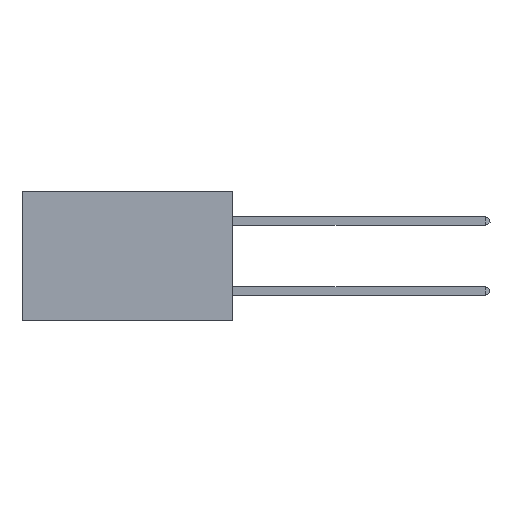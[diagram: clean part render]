
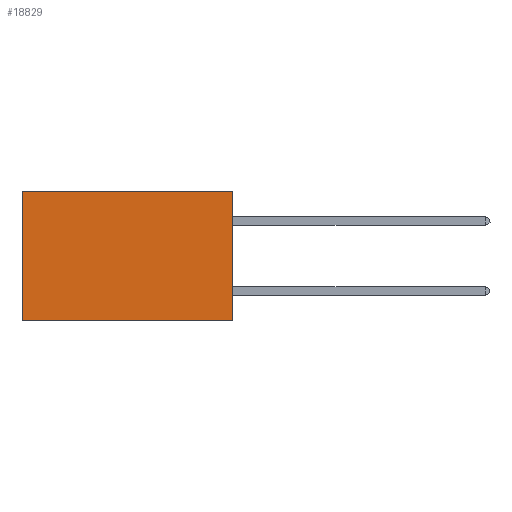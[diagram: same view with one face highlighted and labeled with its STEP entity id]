
A CAD part, left-side view. The second image highlights one B-rep face of the part: STEP entity #18829.
In plain terms, the highlighted planar face has unit normal (-1, 0, 0).
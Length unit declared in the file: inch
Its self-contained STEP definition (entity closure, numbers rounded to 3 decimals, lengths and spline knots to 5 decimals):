
#159 = AXIS2_PLACEMENT_3D ( 'NONE', #17893, #19442, #7616 ) ;
#1968 = LINE ( 'NONE', #11801, #20362 ) ;
#3338 = EDGE_CURVE ( 'NONE', #8968, #4471, #14071, .T. ) ;
#4471 = VERTEX_POINT ( 'NONE', #11150 ) ;
#4704 = DIRECTION ( 'NONE',  ( 0., 0., -1. ) ) ;
#5251 = ORIENTED_EDGE ( 'NONE', *, *, #19631, .T. ) ;
#5755 = ORIENTED_EDGE ( 'NONE', *, *, #20566, .F. ) ;
#6008 = PLANE ( 'NONE',  #159 ) ;
#6185 = CARTESIAN_POINT ( 'NONE',  ( 0.2875, 0., 0. ) ) ;
#6643 = CARTESIAN_POINT ( 'NONE',  ( 0.2875, 0., -0.37 ) ) ;
#6672 = DIRECTION ( 'NONE',  ( 0., 0., -1. ) ) ;
#6883 = VECTOR ( 'NONE', #18465, 39.37008 ) ;
#7099 = ORIENTED_EDGE ( 'NONE', *, *, #9018, .T. ) ;
#7616 = DIRECTION ( 'NONE',  ( 0., 0., -1. ) ) ;
#7889 = CARTESIAN_POINT ( 'NONE',  ( 0.2875, 0.6, 0. ) ) ;
#7959 = VERTEX_POINT ( 'NONE', #7889 ) ;
#7992 = LINE ( 'NONE', #21994, #21029 ) ;
#8968 = VERTEX_POINT ( 'NONE', #10997 ) ;
#9018 = EDGE_CURVE ( 'NONE', #7959, #4471, #7992, .T. ) ;
#10997 = CARTESIAN_POINT ( 'NONE',  ( 0.2875, 0., -0.37 ) ) ;
#11150 = CARTESIAN_POINT ( 'NONE',  ( 0.2875, 0.6, -0.37 ) ) ;
#11801 = CARTESIAN_POINT ( 'NONE',  ( 0.2875, 0., 0. ) ) ;
#12935 = VECTOR ( 'NONE', #21200, 39.37008 ) ;
#14071 = LINE ( 'NONE', #6643, #6883 ) ;
#14883 = FACE_OUTER_BOUND ( 'NONE', #21826, .T. ) ;
#15905 = CARTESIAN_POINT ( 'NONE',  ( 0.2875, 0., 0. ) ) ;
#17784 = LINE ( 'NONE', #15905, #12935 ) ;
#17893 = CARTESIAN_POINT ( 'NONE',  ( 0.2875, 0., 0. ) ) ;
#18003 = ORIENTED_EDGE ( 'NONE', *, *, #3338, .F. ) ;
#18306 = VERTEX_POINT ( 'NONE', #6185 ) ;
#18465 = DIRECTION ( 'NONE',  ( 0., 1., 0. ) ) ;
#18829 = ADVANCED_FACE ( 'NONE', ( #14883 ), #6008, .F. ) ;
#19442 = DIRECTION ( 'NONE',  ( 1., 0., 0. ) ) ;
#19631 = EDGE_CURVE ( 'NONE', #18306, #7959, #17784, .T. ) ;
#20362 = VECTOR ( 'NONE', #6672, 39.37008 ) ;
#20566 = EDGE_CURVE ( 'NONE', #18306, #8968, #1968, .T. ) ;
#21029 = VECTOR ( 'NONE', #4704, 39.37008 ) ;
#21200 = DIRECTION ( 'NONE',  ( 0., 1., 0. ) ) ;
#21826 = EDGE_LOOP ( 'NONE', ( #7099, #18003, #5755, #5251 ) ) ;
#21994 = CARTESIAN_POINT ( 'NONE',  ( 0.2875, 0.6, 0. ) ) ;
